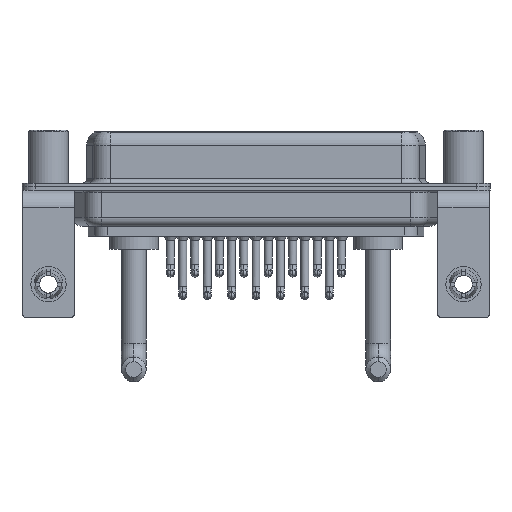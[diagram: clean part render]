
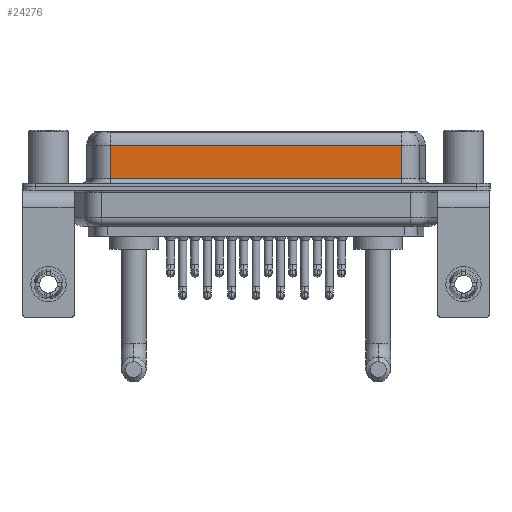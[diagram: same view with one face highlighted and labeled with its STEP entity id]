
A CAD part, front view. The second image highlights one B-rep face of the part: STEP entity #24276.
In plain terms, the highlighted planar face has unit normal (0, -1, 0).
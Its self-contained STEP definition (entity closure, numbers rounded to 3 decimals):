
#144 = LINE ( 'NONE', #24334, #21153 ) ;
#202 = ORIENTED_EDGE ( 'NONE', *, *, #19920, .T. ) ;
#1138 = CARTESIAN_POINT ( 'NONE',  ( 40.037, -3.95, 6.4 ) ) ;
#1414 = CARTESIAN_POINT ( 'NONE',  ( 7.013, -3.95, 4.65 ) ) ;
#1659 = ORIENTED_EDGE ( 'NONE', *, *, #6642, .T. ) ;
#2242 = VECTOR ( 'NONE', #24263, 1000. ) ;
#2847 = CARTESIAN_POINT ( 'NONE',  ( 40.037, -3.95, 0.9 ) ) ;
#4206 = ORIENTED_EDGE ( 'NONE', *, *, #7961, .F. ) ;
#4849 = DIRECTION ( 'NONE',  ( 1., 0., 0. ) ) ;
#5020 = CARTESIAN_POINT ( 'NONE',  ( 40.037, -3.95, 4.65 ) ) ;
#5294 = CARTESIAN_POINT ( 'NONE',  ( 40.037, -3.95, 6.4 ) ) ;
#5545 = DIRECTION ( 'NONE',  ( 0., 0., 1. ) ) ;
#6434 = CARTESIAN_POINT ( 'NONE',  ( 40.037, -3.95, 4.65 ) ) ;
#6642 = EDGE_CURVE ( 'NONE', #7289, #14844, #7256, .T. ) ;
#7256 = LINE ( 'NONE', #5020, #2242 ) ;
#7289 = VERTEX_POINT ( 'NONE', #6434 ) ;
#7961 = EDGE_CURVE ( 'NONE', #7289, #13882, #18062, .T. ) ;
#8684 = DIRECTION ( 'NONE',  ( 0., 0., -1. ) ) ;
#9126 = FACE_OUTER_BOUND ( 'NONE', #11322, .T. ) ;
#9253 = PLANE ( 'NONE',  #21274 ) ;
#11322 = EDGE_LOOP ( 'NONE', ( #4206, #1659, #21427, #202 ) ) ;
#12890 = VECTOR ( 'NONE', #4849, 1000. ) ;
#13882 = VERTEX_POINT ( 'NONE', #2847 ) ;
#13885 = CARTESIAN_POINT ( 'NONE',  ( 7.013, -3.95, 0.9 ) ) ;
#14844 = VERTEX_POINT ( 'NONE', #1414 ) ;
#17466 = VECTOR ( 'NONE', #8684, 1000. ) ;
#18062 = LINE ( 'NONE', #1138, #17466 ) ;
#18304 = CARTESIAN_POINT ( 'NONE',  ( 40.037, -3.95, 0.9 ) ) ;
#18908 = DIRECTION ( 'NONE',  ( 0., 0., -1. ) ) ;
#19920 = EDGE_CURVE ( 'NONE', #23113, #13882, #20023, .T. ) ;
#20023 = LINE ( 'NONE', #18304, #12890 ) ;
#20067 = EDGE_CURVE ( 'NONE', #14844, #23113, #144, .T. ) ;
#21153 = VECTOR ( 'NONE', #18908, 1000. ) ;
#21274 = AXIS2_PLACEMENT_3D ( 'NONE', #5294, #24177, #5545 ) ;
#21427 = ORIENTED_EDGE ( 'NONE', *, *, #20067, .T. ) ;
#23113 = VERTEX_POINT ( 'NONE', #13885 ) ;
#24177 = DIRECTION ( 'NONE',  ( 0., 1., 0. ) ) ;
#24263 = DIRECTION ( 'NONE',  ( -1., 0., 0. ) ) ;
#24276 = ADVANCED_FACE ( 'NONE', ( #9126 ), #9253, .F. ) ;
#24334 = CARTESIAN_POINT ( 'NONE',  ( 7.013, -3.95, 6.4 ) ) ;
